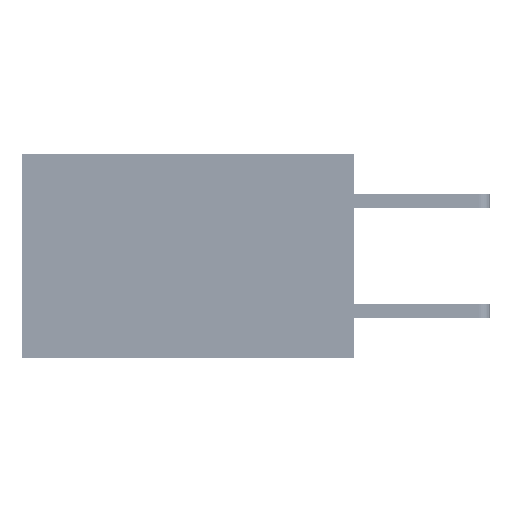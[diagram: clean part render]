
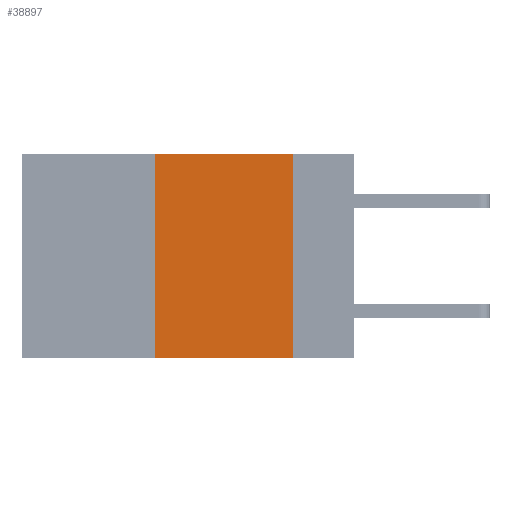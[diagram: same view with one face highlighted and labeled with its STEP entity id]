
A CAD part, left-side view. The second image highlights one B-rep face of the part: STEP entity #38897.
In plain terms, the highlighted planar face has unit normal (-1, 0, 0).
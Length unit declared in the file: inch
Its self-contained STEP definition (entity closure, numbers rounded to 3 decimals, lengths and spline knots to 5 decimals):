
#355 = EDGE_CURVE ( 'NONE', #35822, #30978, #21380, .T. ) ;
#645 = CARTESIAN_POINT ( 'NONE',  ( 0., 0.36, -0.37 ) ) ;
#851 = VECTOR ( 'NONE', #27525, 39.37008 ) ;
#1374 = DIRECTION ( 'NONE',  ( 1., 0., 0. ) ) ;
#1580 = FACE_OUTER_BOUND ( 'NONE', #4127, .T. ) ;
#2120 = VECTOR ( 'NONE', #14921, 39.37008 ) ;
#2946 = AXIS2_PLACEMENT_3D ( 'NONE', #17400, #1374, #29960 ) ;
#2983 = EDGE_CURVE ( 'NONE', #35822, #39260, #8967, .T. ) ;
#4127 = EDGE_LOOP ( 'NONE', ( #33076, #30115, #21485, #37872 ) ) ;
#7768 = LINE ( 'NONE', #38827, #37556 ) ;
#8223 = VECTOR ( 'NONE', #27150, 39.37008 ) ;
#8967 = LINE ( 'NONE', #23988, #2120 ) ;
#10170 = CARTESIAN_POINT ( 'NONE',  ( 0., 0.11, -0.37 ) ) ;
#11562 = CARTESIAN_POINT ( 'NONE',  ( 0., 0.36, 0. ) ) ;
#13320 = EDGE_CURVE ( 'NONE', #30978, #24122, #7768, .T. ) ;
#14921 = DIRECTION ( 'NONE',  ( 0., -1., 0. ) ) ;
#16591 = DIRECTION ( 'NONE',  ( 0., -1., 0. ) ) ;
#17400 = CARTESIAN_POINT ( 'NONE',  ( 0., 0.6, 0. ) ) ;
#17656 = LINE ( 'NONE', #24631, #851 ) ;
#18669 = EDGE_CURVE ( 'NONE', #24122, #39260, #17656, .T. ) ;
#21380 = LINE ( 'NONE', #37424, #8223 ) ;
#21485 = ORIENTED_EDGE ( 'NONE', *, *, #355, .F. ) ;
#23988 = CARTESIAN_POINT ( 'NONE',  ( 0., 0.6, -0.37 ) ) ;
#24122 = VERTEX_POINT ( 'NONE', #33137 ) ;
#24631 = CARTESIAN_POINT ( 'NONE',  ( 0., 0.11, 0. ) ) ;
#27150 = DIRECTION ( 'NONE',  ( 0., 0., 1. ) ) ;
#27525 = DIRECTION ( 'NONE',  ( 0., 0., -1. ) ) ;
#29960 = DIRECTION ( 'NONE',  ( 0., 0., -1. ) ) ;
#30115 = ORIENTED_EDGE ( 'NONE', *, *, #13320, .F. ) ;
#30160 = PLANE ( 'NONE',  #2946 ) ;
#30978 = VERTEX_POINT ( 'NONE', #11562 ) ;
#33076 = ORIENTED_EDGE ( 'NONE', *, *, #18669, .F. ) ;
#33137 = CARTESIAN_POINT ( 'NONE',  ( 0., 0.11, 0. ) ) ;
#35822 = VERTEX_POINT ( 'NONE', #645 ) ;
#37424 = CARTESIAN_POINT ( 'NONE',  ( 0., 0.36, 0. ) ) ;
#37556 = VECTOR ( 'NONE', #16591, 39.37008 ) ;
#37872 = ORIENTED_EDGE ( 'NONE', *, *, #2983, .T. ) ;
#38827 = CARTESIAN_POINT ( 'NONE',  ( 0., 0.6, 0. ) ) ;
#38897 = ADVANCED_FACE ( 'NONE', ( #1580 ), #30160, .F. ) ;
#39260 = VERTEX_POINT ( 'NONE', #10170 ) ;
